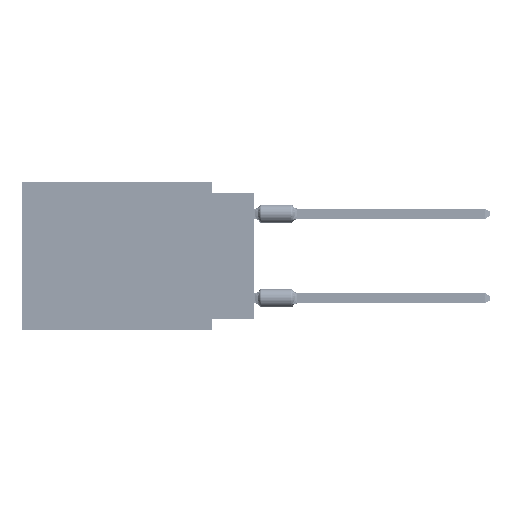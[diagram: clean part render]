
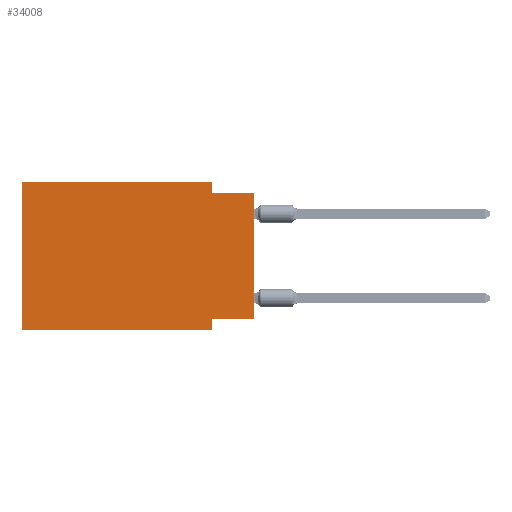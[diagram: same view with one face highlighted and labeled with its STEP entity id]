
A CAD part, left-side view. The second image highlights one B-rep face of the part: STEP entity #34008.
In plain terms, the highlighted planar face has unit normal (-1, 0, 0).
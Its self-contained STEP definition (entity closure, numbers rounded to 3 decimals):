
#32 = FACE_OUTER_BOUND ( 'NONE', #19326, .T. ) ;
#607 = CARTESIAN_POINT ( 'NONE',  ( 0., 2.54, -8.89 ) ) ;
#1927 = LINE ( 'NONE', #58373, #17356 ) ;
#2697 = CARTESIAN_POINT ( 'NONE',  ( 0., 13.97, 0. ) ) ;
#3206 = ORIENTED_EDGE ( 'NONE', *, *, #45465, .F. ) ;
#3253 = VECTOR ( 'NONE', #10642, 1000. ) ;
#3468 = DIRECTION ( 'NONE',  ( 0., -1., 0. ) ) ;
#5442 = LINE ( 'NONE', #25831, #41536 ) ;
#7889 = VERTEX_POINT ( 'NONE', #49167 ) ;
#9568 = EDGE_CURVE ( 'NONE', #64372, #44360, #65804, .T. ) ;
#9970 = LINE ( 'NONE', #40658, #45055 ) ;
#10642 = DIRECTION ( 'NONE',  ( 0., 0., 1. ) ) ;
#11914 = VECTOR ( 'NONE', #20973, 1000. ) ;
#14145 = CARTESIAN_POINT ( 'NONE',  ( 0., 13.97, -8.89 ) ) ;
#14246 = VERTEX_POINT ( 'NONE', #59527 ) ;
#16299 = DIRECTION ( 'NONE',  ( 0., 0., -1. ) ) ;
#16946 = ORIENTED_EDGE ( 'NONE', *, *, #9568, .T. ) ;
#17356 = VECTOR ( 'NONE', #17951, 1000. ) ;
#17951 = DIRECTION ( 'NONE',  ( 0., 1., 0. ) ) ;
#18397 = EDGE_CURVE ( 'NONE', #41639, #7889, #37759, .T. ) ;
#19326 = EDGE_LOOP ( 'NONE', ( #16946, #38956, #3206, #63300, #33621, #34583, #26787, #42950 ) ) ;
#20419 = CARTESIAN_POINT ( 'NONE',  ( 0., 13.97, 0. ) ) ;
#20973 = DIRECTION ( 'NONE',  ( 0., 0., -1. ) ) ;
#22642 = CARTESIAN_POINT ( 'NONE',  ( 0., 13.97, 0. ) ) ;
#22764 = VERTEX_POINT ( 'NONE', #24632 ) ;
#23696 = CARTESIAN_POINT ( 'NONE',  ( 0., 13.97, 0. ) ) ;
#24632 = CARTESIAN_POINT ( 'NONE',  ( 0., 2.54, -8.255 ) ) ;
#25831 = CARTESIAN_POINT ( 'NONE',  ( 0., 0., -0.635 ) ) ;
#26036 = EDGE_CURVE ( 'NONE', #58104, #44360, #5442, .T. ) ;
#26787 = ORIENTED_EDGE ( 'NONE', *, *, #31610, .F. ) ;
#27633 = VECTOR ( 'NONE', #3468, 1000. ) ;
#28511 = CARTESIAN_POINT ( 'NONE',  ( 0., 2.54, -0.635 ) ) ;
#30253 = AXIS2_PLACEMENT_3D ( 'NONE', #20419, #49818, #65198 ) ;
#31610 = EDGE_CURVE ( 'NONE', #22764, #14246, #56708, .T. ) ;
#32885 = EDGE_CURVE ( 'NONE', #64372, #22764, #1927, .T. ) ;
#33621 = ORIENTED_EDGE ( 'NONE', *, *, #52650, .F. ) ;
#34008 = ADVANCED_FACE ( 'NONE', ( #32 ), #60525, .F. ) ;
#34583 = ORIENTED_EDGE ( 'NONE', *, *, #59703, .T. ) ;
#35533 = VECTOR ( 'NONE', #43414, 1000. ) ;
#35716 = CARTESIAN_POINT ( 'NONE',  ( 0., 0., 0. ) ) ;
#37759 = LINE ( 'NONE', #2697, #35533 ) ;
#37989 = DIRECTION ( 'NONE',  ( 0., 0., 1. ) ) ;
#38956 = ORIENTED_EDGE ( 'NONE', *, *, #26036, .F. ) ;
#39512 = DIRECTION ( 'NONE',  ( 0., -1., 0. ) ) ;
#40658 = CARTESIAN_POINT ( 'NONE',  ( 0., 2.54, 0. ) ) ;
#41536 = VECTOR ( 'NONE', #39512, 1000. ) ;
#41639 = VERTEX_POINT ( 'NONE', #23696 ) ;
#42950 = ORIENTED_EDGE ( 'NONE', *, *, #32885, .F. ) ;
#43414 = DIRECTION ( 'NONE',  ( 0., -1., 0. ) ) ;
#44360 = VERTEX_POINT ( 'NONE', #49211 ) ;
#45055 = VECTOR ( 'NONE', #16299, 1000. ) ;
#45465 = EDGE_CURVE ( 'NONE', #7889, #58104, #9970, .T. ) ;
#47218 = VECTOR ( 'NONE', #37989, 1000. ) ;
#47365 = LINE ( 'NONE', #22642, #47218 ) ;
#49167 = CARTESIAN_POINT ( 'NONE',  ( 0., 2.54, 0. ) ) ;
#49211 = CARTESIAN_POINT ( 'NONE',  ( 0., 0., -0.635 ) ) ;
#49818 = DIRECTION ( 'NONE',  ( 1., 0., 0. ) ) ;
#52247 = CARTESIAN_POINT ( 'NONE',  ( 0., 13.97, -8.89 ) ) ;
#52650 = EDGE_CURVE ( 'NONE', #57881, #41639, #47365, .T. ) ;
#56708 = LINE ( 'NONE', #607, #11914 ) ;
#57881 = VERTEX_POINT ( 'NONE', #52247 ) ;
#58104 = VERTEX_POINT ( 'NONE', #28511 ) ;
#58373 = CARTESIAN_POINT ( 'NONE',  ( 0., 0., -8.255 ) ) ;
#59527 = CARTESIAN_POINT ( 'NONE',  ( 0., 2.54, -8.89 ) ) ;
#59703 = EDGE_CURVE ( 'NONE', #57881, #14246, #65587, .T. ) ;
#59817 = CARTESIAN_POINT ( 'NONE',  ( 0., 0., -8.255 ) ) ;
#60525 = PLANE ( 'NONE',  #30253 ) ;
#63300 = ORIENTED_EDGE ( 'NONE', *, *, #18397, .F. ) ;
#64372 = VERTEX_POINT ( 'NONE', #59817 ) ;
#65198 = DIRECTION ( 'NONE',  ( 0., 0., -1. ) ) ;
#65587 = LINE ( 'NONE', #14145, #27633 ) ;
#65804 = LINE ( 'NONE', #35716, #3253 ) ;
